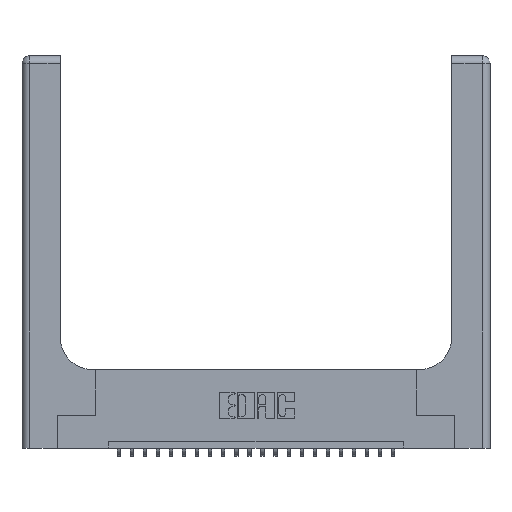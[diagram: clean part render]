
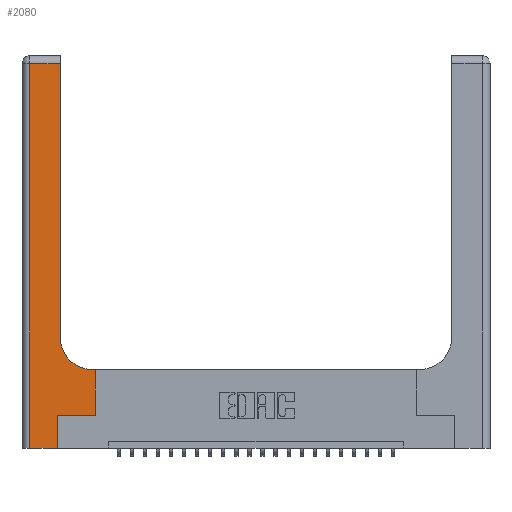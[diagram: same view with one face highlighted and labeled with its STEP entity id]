
A CAD part, top view. The second image highlights one B-rep face of the part: STEP entity #2080.
In plain terms, the highlighted planar face has unit normal (0, 0, 1).
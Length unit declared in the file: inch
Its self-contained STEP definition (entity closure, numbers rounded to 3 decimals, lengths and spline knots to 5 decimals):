
#130 = AXIS2_PLACEMENT_3D ( 'NONE', #15777, #19318, #19484 ) ;
#190 = DIRECTION ( 'NONE',  ( 0., 1., 0. ) ) ;
#851 = VECTOR ( 'NONE', #11436, 39.37008 ) ;
#1184 = DIRECTION ( 'NONE',  ( 0., -1., 0. ) ) ;
#2080 = ADVANCED_FACE ( 'NONE', ( #14500 ), #6172, .F. ) ;
#2301 = LINE ( 'NONE', #5461, #851 ) ;
#2572 = CARTESIAN_POINT ( 'NONE',  ( 0.5585, 0.25, 0.37 ) ) ;
#2584 = ORIENTED_EDGE ( 'NONE', *, *, #14240, .T. ) ;
#2600 = ORIENTED_EDGE ( 'NONE', *, *, #15163, .T. ) ;
#2857 = CARTESIAN_POINT ( 'NONE',  ( 0.5585, 0.6, 0.37 ) ) ;
#2915 = LINE ( 'NONE', #17700, #15093 ) ;
#3673 = LINE ( 'NONE', #19471, #11113 ) ;
#4284 = LINE ( 'NONE', #5061, #9922 ) ;
#4922 = EDGE_CURVE ( 'NONE', #5558, #23887, #4284, .T. ) ;
#5061 = CARTESIAN_POINT ( 'NONE',  ( 0.06, 3., 0.37 ) ) ;
#5233 = EDGE_CURVE ( 'NONE', #18515, #20080, #21226, .T. ) ;
#5426 = ORIENTED_EDGE ( 'NONE', *, *, #13302, .T. ) ;
#5461 = CARTESIAN_POINT ( 'NONE',  ( 0., 2.94, 0.37 ) ) ;
#5558 = VERTEX_POINT ( 'NONE', #15892 ) ;
#6172 = PLANE ( 'NONE',  #130 ) ;
#7763 = ORIENTED_EDGE ( 'NONE', *, *, #19742, .T. ) ;
#8079 = DIRECTION ( 'NONE',  ( 1., 0., 0. ) ) ;
#8452 = DIRECTION ( 'NONE',  ( 0., 1., 0. ) ) ;
#8619 = CARTESIAN_POINT ( 'NONE',  ( 0.5585, 0.25, 0.37 ) ) ;
#8704 = CARTESIAN_POINT ( 'NONE',  ( 0.5415, 0.85, 0.37 ) ) ;
#8901 = ORIENTED_EDGE ( 'NONE', *, *, #13725, .T. ) ;
#9376 = LINE ( 'NONE', #9410, #18304 ) ;
#9410 = CARTESIAN_POINT ( 'NONE',  ( 0.269, 0., 0.37 ) ) ;
#9522 = ORIENTED_EDGE ( 'NONE', *, *, #4922, .T. ) ;
#9922 = VECTOR ( 'NONE', #1184, 39.37008 ) ;
#10188 = VERTEX_POINT ( 'NONE', #2857 ) ;
#11113 = VECTOR ( 'NONE', #8079, 39.37008 ) ;
#11436 = DIRECTION ( 'NONE',  ( -1., 0., 0. ) ) ;
#11924 = VERTEX_POINT ( 'NONE', #14640 ) ;
#12532 = DIRECTION ( 'NONE',  ( 1., 0., 0. ) ) ;
#12897 = EDGE_CURVE ( 'NONE', #16233, #10188, #19569, .T. ) ;
#13231 = VERTEX_POINT ( 'NONE', #20860 ) ;
#13273 = ORIENTED_EDGE ( 'NONE', *, *, #22781, .T. ) ;
#13302 = EDGE_CURVE ( 'NONE', #20080, #13231, #2915, .T. ) ;
#13457 = CARTESIAN_POINT ( 'NONE',  ( 0.5415, 0.6, 0.37 ) ) ;
#13725 = EDGE_CURVE ( 'NONE', #13231, #5558, #2301, .T. ) ;
#13810 = DIRECTION ( 'NONE',  ( 0., 1., 0. ) ) ;
#14240 = EDGE_CURVE ( 'NONE', #18111, #11924, #9376, .T. ) ;
#14500 = FACE_OUTER_BOUND ( 'NONE', #23236, .T. ) ;
#14640 = CARTESIAN_POINT ( 'NONE',  ( 0.269, 0.25, 0.37 ) ) ;
#15082 = CARTESIAN_POINT ( 'NONE',  ( 0., 0., 0.37 ) ) ;
#15093 = VECTOR ( 'NONE', #13810, 39.37008 ) ;
#15163 = EDGE_CURVE ( 'NONE', #23887, #18111, #15281, .T. ) ;
#15281 = LINE ( 'NONE', #15082, #20026 ) ;
#15305 = CARTESIAN_POINT ( 'NONE',  ( 0.2915, 0.6, 0.37 ) ) ;
#15777 = CARTESIAN_POINT ( 'NONE',  ( 0., 3., 0.37 ) ) ;
#15892 = CARTESIAN_POINT ( 'NONE',  ( 0.06, 2.94, 0.37 ) ) ;
#16233 = VERTEX_POINT ( 'NONE', #2572 ) ;
#16902 = DIRECTION ( 'NONE',  ( 1., 0., 0. ) ) ;
#17204 = ORIENTED_EDGE ( 'NONE', *, *, #5233, .T. ) ;
#17700 = CARTESIAN_POINT ( 'NONE',  ( 0.2915, 3., 0.37 ) ) ;
#18111 = VERTEX_POINT ( 'NONE', #19466 ) ;
#18304 = VECTOR ( 'NONE', #190, 39.37008 ) ;
#18346 = CARTESIAN_POINT ( 'NONE',  ( 0.06, 0., 0.37 ) ) ;
#18515 = VERTEX_POINT ( 'NONE', #13457 ) ;
#18982 = LINE ( 'NONE', #15305, #24281 ) ;
#19318 = DIRECTION ( 'NONE',  ( 0., 0., -1. ) ) ;
#19466 = CARTESIAN_POINT ( 'NONE',  ( 0.269, 0., 0.37 ) ) ;
#19471 = CARTESIAN_POINT ( 'NONE',  ( 0.269, 0.25, 0.37 ) ) ;
#19484 = DIRECTION ( 'NONE',  ( -1., 0., 0. ) ) ;
#19569 = LINE ( 'NONE', #8619, #20451 ) ;
#19742 = EDGE_CURVE ( 'NONE', #10188, #18515, #18982, .T. ) ;
#20001 = AXIS2_PLACEMENT_3D ( 'NONE', #8704, #23859, #12532 ) ;
#20026 = VECTOR ( 'NONE', #16902, 39.37008 ) ;
#20080 = VERTEX_POINT ( 'NONE', #22501 ) ;
#20451 = VECTOR ( 'NONE', #8452, 39.37008 ) ;
#20584 = ORIENTED_EDGE ( 'NONE', *, *, #12897, .T. ) ;
#20860 = CARTESIAN_POINT ( 'NONE',  ( 0.2915, 2.94, 0.37 ) ) ;
#21226 = CIRCLE ( 'NONE', #20001, 0.25 ) ;
#22501 = CARTESIAN_POINT ( 'NONE',  ( 0.2915, 0.85, 0.37 ) ) ;
#22781 = EDGE_CURVE ( 'NONE', #11924, #16233, #3673, .T. ) ;
#22912 = DIRECTION ( 'NONE',  ( -1., 0., 0. ) ) ;
#23236 = EDGE_LOOP ( 'NONE', ( #5426, #8901, #9522, #2600, #2584, #13273, #20584, #7763, #17204 ) ) ;
#23859 = DIRECTION ( 'NONE',  ( 0., 0., -1. ) ) ;
#23887 = VERTEX_POINT ( 'NONE', #18346 ) ;
#24281 = VECTOR ( 'NONE', #22912, 39.37008 ) ;
